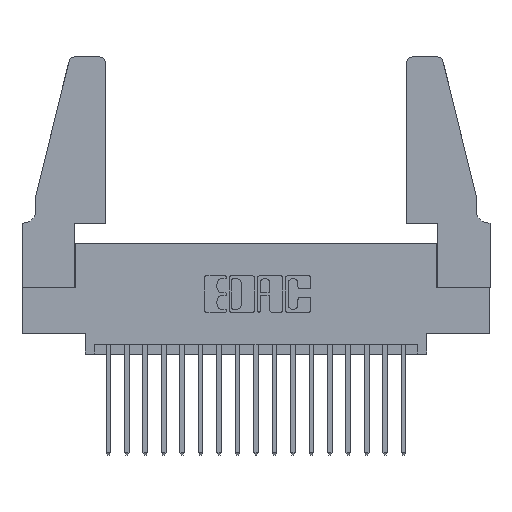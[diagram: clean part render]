
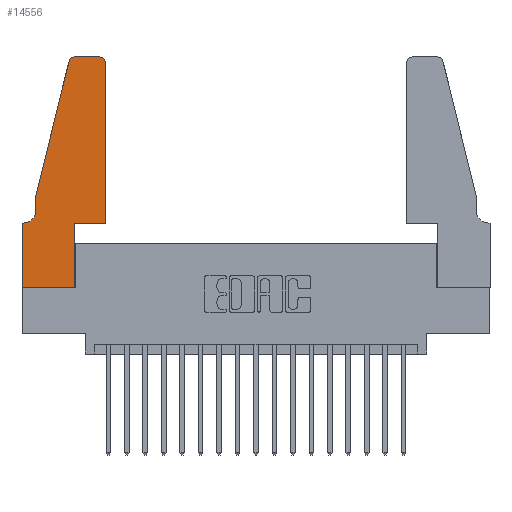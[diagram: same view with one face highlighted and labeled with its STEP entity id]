
A CAD part, top view. The second image highlights one B-rep face of the part: STEP entity #14556.
In plain terms, the highlighted planar face has unit normal (0, 0, 1).
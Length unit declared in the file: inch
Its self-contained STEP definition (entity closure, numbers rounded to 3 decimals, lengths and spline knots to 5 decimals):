
#33 = EDGE_CURVE ( 'NONE', #16121, #10863, #16320, .T. ) ;
#155 = DIRECTION ( 'NONE',  ( 1., 0., 0. ) ) ;
#178 = VERTEX_POINT ( 'NONE', #6455 ) ;
#195 = EDGE_CURVE ( 'NONE', #10863, #937, #10131, .T. ) ;
#278 = ORIENTED_EDGE ( 'NONE', *, *, #9843, .T. ) ;
#373 = VERTEX_POINT ( 'NONE', #3385 ) ;
#594 = LINE ( 'NONE', #18593, #2658 ) ;
#934 = VECTOR ( 'NONE', #16923, 39.37008 ) ;
#937 = VERTEX_POINT ( 'NONE', #12239 ) ;
#1534 = AXIS2_PLACEMENT_3D ( 'NONE', #14648, #2704, #18938 ) ;
#1551 = EDGE_CURVE ( 'NONE', #19029, #4043, #11220, .T. ) ;
#2077 = DIRECTION ( 'NONE',  ( -1., 0., 0. ) ) ;
#2531 = PLANE ( 'NONE',  #1534 ) ;
#2543 = EDGE_CURVE ( 'NONE', #8946, #16121, #6588, .T. ) ;
#2593 = EDGE_CURVE ( 'NONE', #7369, #8946, #12781, .T. ) ;
#2658 = VECTOR ( 'NONE', #15757, 39.37008 ) ;
#2690 = CARTESIAN_POINT ( 'NONE',  ( 0.0755, 0.5, 0.37 ) ) ;
#2704 = DIRECTION ( 'NONE',  ( 0., 0., 1. ) ) ;
#2781 = DIRECTION ( 'NONE',  ( 0., 1., 0. ) ) ;
#3099 = CARTESIAN_POINT ( 'NONE',  ( 0.2865, 0., 0.37 ) ) ;
#3193 = ORIENTED_EDGE ( 'NONE', *, *, #2593, .T. ) ;
#3385 = CARTESIAN_POINT ( 'NONE',  ( 0., 0.35, 0.37 ) ) ;
#3408 = EDGE_CURVE ( 'NONE', #4043, #178, #594, .T. ) ;
#4043 = VERTEX_POINT ( 'NONE', #10999 ) ;
#4044 = CARTESIAN_POINT ( 'NONE',  ( 0.4205, 1.22, 0.37 ) ) ;
#4097 = CARTESIAN_POINT ( 'NONE',  ( 0.4505, 0.35, 0.37 ) ) ;
#4231 = DIRECTION ( 'NONE',  ( 1., 0., 0. ) ) ;
#4426 = CARTESIAN_POINT ( 'NONE',  ( 0., 0., 0.37 ) ) ;
#4487 = CARTESIAN_POINT ( 'NONE',  ( 0.4505, 0.35, 0.37 ) ) ;
#5090 = VECTOR ( 'NONE', #10826, 39.37008 ) ;
#5527 = AXIS2_PLACEMENT_3D ( 'NONE', #4044, #5560, #4231 ) ;
#5560 = DIRECTION ( 'NONE',  ( 0., 0., 1. ) ) ;
#6054 = DIRECTION ( 'NONE',  ( -1., 0., 0. ) ) ;
#6455 = CARTESIAN_POINT ( 'NONE',  ( 0.0755, 0.42, 0.37 ) ) ;
#6588 = LINE ( 'NONE', #6655, #13022 ) ;
#6633 = CARTESIAN_POINT ( 'NONE',  ( 0., 0., 0.37 ) ) ;
#6655 = CARTESIAN_POINT ( 'NONE',  ( 0.4505, 0.35, 0.37 ) ) ;
#6697 = VECTOR ( 'NONE', #6054, 39.37008 ) ;
#6960 = CARTESIAN_POINT ( 'NONE',  ( 0.25487, 1.22718, 0.37 ) ) ;
#7100 = EDGE_CURVE ( 'NONE', #373, #13171, #12396, .T. ) ;
#7149 = EDGE_CURVE ( 'NONE', #13171, #7369, #15376, .T. ) ;
#7369 = VERTEX_POINT ( 'NONE', #3099 ) ;
#7628 = VERTEX_POINT ( 'NONE', #12535 ) ;
#7870 = VERTEX_POINT ( 'NONE', #11992 ) ;
#7972 = CIRCLE ( 'NONE', #11424, 0.07 ) ;
#8285 = LINE ( 'NONE', #14917, #6697 ) ;
#8378 = EDGE_CURVE ( 'NONE', #178, #7628, #7972, .T. ) ;
#8822 = DIRECTION ( 'NONE',  ( 1., 0., 0. ) ) ;
#8946 = VERTEX_POINT ( 'NONE', #13166 ) ;
#8949 = VECTOR ( 'NONE', #16223, 39.37008 ) ;
#8965 = LINE ( 'NONE', #12343, #5090 ) ;
#8999 = CARTESIAN_POINT ( 'NONE',  ( 0.284, 1.22, 0.37 ) ) ;
#9358 = DIRECTION ( 'NONE',  ( 0., 0., -1. ) ) ;
#9646 = DIRECTION ( 'NONE',  ( 1., 0., 0. ) ) ;
#9843 = EDGE_CURVE ( 'NONE', #7870, #19029, #18522, .T. ) ;
#9888 = ORIENTED_EDGE ( 'NONE', *, *, #195, .T. ) ;
#9931 = ORIENTED_EDGE ( 'NONE', *, *, #7100, .T. ) ;
#10091 = ORIENTED_EDGE ( 'NONE', *, *, #2543, .T. ) ;
#10131 = CIRCLE ( 'NONE', #5527, 0.03 ) ;
#10392 = ORIENTED_EDGE ( 'NONE', *, *, #33, .T. ) ;
#10439 = FACE_OUTER_BOUND ( 'NONE', #15080, .T. ) ;
#10497 = DIRECTION ( 'NONE',  ( 0., 0., 1. ) ) ;
#10637 = ORIENTED_EDGE ( 'NONE', *, *, #16313, .T. ) ;
#10826 = DIRECTION ( 'NONE',  ( -1., 0., 0. ) ) ;
#10863 = VERTEX_POINT ( 'NONE', #15862 ) ;
#10999 = CARTESIAN_POINT ( 'NONE',  ( 0.0755, 0.5, 0.37 ) ) ;
#11220 = LINE ( 'NONE', #2690, #16031 ) ;
#11424 = AXIS2_PLACEMENT_3D ( 'NONE', #12390, #9358, #2077 ) ;
#11630 = VECTOR ( 'NONE', #2781, 39.37008 ) ;
#11992 = CARTESIAN_POINT ( 'NONE',  ( 0.284, 1.25, 0.37 ) ) ;
#12099 = ORIENTED_EDGE ( 'NONE', *, *, #8378, .T. ) ;
#12239 = CARTESIAN_POINT ( 'NONE',  ( 0.4205, 1.25, 0.37 ) ) ;
#12343 = CARTESIAN_POINT ( 'NONE',  ( 0.0755, 0.35, 0.37 ) ) ;
#12390 = CARTESIAN_POINT ( 'NONE',  ( 0.0055, 0.42, 0.37 ) ) ;
#12396 = LINE ( 'NONE', #6633, #934 ) ;
#12535 = CARTESIAN_POINT ( 'NONE',  ( 0.0055, 0.35, 0.37 ) ) ;
#12542 = AXIS2_PLACEMENT_3D ( 'NONE', #8999, #10497, #155 ) ;
#12752 = ORIENTED_EDGE ( 'NONE', *, *, #16458, .T. ) ;
#12781 = LINE ( 'NONE', #13234, #11630 ) ;
#13022 = VECTOR ( 'NONE', #9646, 39.37008 ) ;
#13127 = ORIENTED_EDGE ( 'NONE', *, *, #1551, .T. ) ;
#13166 = CARTESIAN_POINT ( 'NONE',  ( 0.2865, 0.35, 0.37 ) ) ;
#13171 = VERTEX_POINT ( 'NONE', #14495 ) ;
#13234 = CARTESIAN_POINT ( 'NONE',  ( 0.2865, 0.35, 0.37 ) ) ;
#14434 = DIRECTION ( 'NONE',  ( -0.239, -0.971, 0. ) ) ;
#14495 = CARTESIAN_POINT ( 'NONE',  ( 0., 0., 0.37 ) ) ;
#14556 = ADVANCED_FACE ( 'NONE', ( #10439 ), #2531, .T. ) ;
#14648 = CARTESIAN_POINT ( 'NONE',  ( 0., 0.35, 0.37 ) ) ;
#14917 = CARTESIAN_POINT ( 'NONE',  ( 0.2605, 1.25, 0.37 ) ) ;
#15080 = EDGE_LOOP ( 'NONE', ( #10637, #278, #13127, #16914, #12099, #12752, #9931, #18349, #3193, #10091, #10392, #9888 ) ) ;
#15376 = LINE ( 'NONE', #4426, #16062 ) ;
#15757 = DIRECTION ( 'NONE',  ( 0., -1., 0. ) ) ;
#15862 = CARTESIAN_POINT ( 'NONE',  ( 0.4505, 1.22, 0.37 ) ) ;
#16031 = VECTOR ( 'NONE', #14434, 39.37008 ) ;
#16062 = VECTOR ( 'NONE', #8822, 39.37008 ) ;
#16121 = VERTEX_POINT ( 'NONE', #4097 ) ;
#16223 = DIRECTION ( 'NONE',  ( 0., 1., 0. ) ) ;
#16313 = EDGE_CURVE ( 'NONE', #937, #7870, #8285, .T. ) ;
#16320 = LINE ( 'NONE', #4487, #8949 ) ;
#16458 = EDGE_CURVE ( 'NONE', #7628, #373, #8965, .T. ) ;
#16914 = ORIENTED_EDGE ( 'NONE', *, *, #3408, .T. ) ;
#16923 = DIRECTION ( 'NONE',  ( 0., -1., 0. ) ) ;
#18349 = ORIENTED_EDGE ( 'NONE', *, *, #7149, .T. ) ;
#18522 = CIRCLE ( 'NONE', #12542, 0.03 ) ;
#18593 = CARTESIAN_POINT ( 'NONE',  ( 0.0755, 0.5, 0.37 ) ) ;
#18938 = DIRECTION ( 'NONE',  ( 1., 0., 0. ) ) ;
#19029 = VERTEX_POINT ( 'NONE', #6960 ) ;
